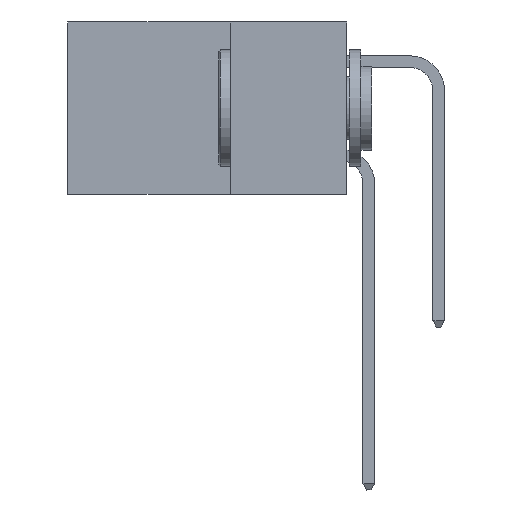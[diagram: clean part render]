
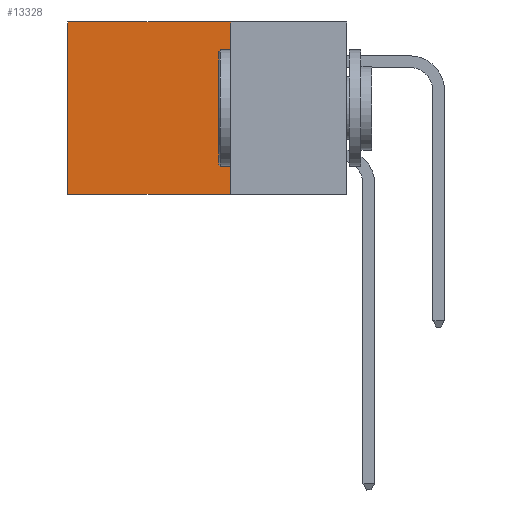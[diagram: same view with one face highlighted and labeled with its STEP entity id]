
A CAD part, left-side view. The second image highlights one B-rep face of the part: STEP entity #13328.
In plain terms, the highlighted planar face has unit normal (-1, 0, 0).
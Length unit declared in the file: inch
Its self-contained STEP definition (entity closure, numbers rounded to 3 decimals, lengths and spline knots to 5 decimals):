
#483 = ORIENTED_EDGE ( 'NONE', *, *, #14786, .F. ) ;
#1495 = CARTESIAN_POINT ( 'NONE',  ( 0.2875, 0.25, 0. ) ) ;
#2049 = ORIENTED_EDGE ( 'NONE', *, *, #6741, .F. ) ;
#3182 = CARTESIAN_POINT ( 'NONE',  ( 0.2875, 0.6, 0. ) ) ;
#3629 = DIRECTION ( 'NONE',  ( 0., 0., -1. ) ) ;
#5018 = VERTEX_POINT ( 'NONE', #12438 ) ;
#5411 = DIRECTION ( 'NONE',  ( 0., 0., -1. ) ) ;
#5612 = EDGE_LOOP ( 'NONE', ( #24950, #483, #2049, #9877 ) ) ;
#6403 = LINE ( 'NONE', #14993, #26133 ) ;
#6741 = EDGE_CURVE ( 'NONE', #13102, #5018, #8214, .T. ) ;
#6752 = DIRECTION ( 'NONE',  ( 0., 1., 0. ) ) ;
#8214 = LINE ( 'NONE', #10666, #30839 ) ;
#9877 = ORIENTED_EDGE ( 'NONE', *, *, #10642, .T. ) ;
#10642 = EDGE_CURVE ( 'NONE', #13102, #13510, #6403, .T. ) ;
#10666 = CARTESIAN_POINT ( 'NONE',  ( 0.2875, 0.25, 0. ) ) ;
#10961 = CARTESIAN_POINT ( 'NONE',  ( 0.2875, 0.6, -0.37 ) ) ;
#12245 = CARTESIAN_POINT ( 'NONE',  ( 0.2875, 0.25, 0. ) ) ;
#12438 = CARTESIAN_POINT ( 'NONE',  ( 0.2875, 0.25, -0.37 ) ) ;
#13102 = VERTEX_POINT ( 'NONE', #12245 ) ;
#13328 = ADVANCED_FACE ( 'NONE', ( #21765 ), #22157, .F. ) ;
#13510 = VERTEX_POINT ( 'NONE', #21050 ) ;
#13900 = DIRECTION ( 'NONE',  ( 1., 0., 0. ) ) ;
#13992 = VECTOR ( 'NONE', #24075, 39.37008 ) ;
#14786 = EDGE_CURVE ( 'NONE', #5018, #24750, #23316, .T. ) ;
#14993 = CARTESIAN_POINT ( 'NONE',  ( 0.2875, 0.25, 0. ) ) ;
#21050 = CARTESIAN_POINT ( 'NONE',  ( 0.2875, 0.6, 0. ) ) ;
#21234 = DIRECTION ( 'NONE',  ( 0., 0., -1. ) ) ;
#21765 = FACE_OUTER_BOUND ( 'NONE', #5612, .T. ) ;
#22157 = PLANE ( 'NONE',  #28763 ) ;
#23316 = LINE ( 'NONE', #31702, #13992 ) ;
#23651 = VECTOR ( 'NONE', #21234, 39.37008 ) ;
#24075 = DIRECTION ( 'NONE',  ( 0., 1., 0. ) ) ;
#24750 = VERTEX_POINT ( 'NONE', #10961 ) ;
#24950 = ORIENTED_EDGE ( 'NONE', *, *, #30598, .T. ) ;
#26133 = VECTOR ( 'NONE', #6752, 39.37008 ) ;
#28763 = AXIS2_PLACEMENT_3D ( 'NONE', #1495, #13900, #3629 ) ;
#30504 = LINE ( 'NONE', #3182, #23651 ) ;
#30598 = EDGE_CURVE ( 'NONE', #13510, #24750, #30504, .T. ) ;
#30839 = VECTOR ( 'NONE', #5411, 39.37008 ) ;
#31702 = CARTESIAN_POINT ( 'NONE',  ( 0.2875, 0.25, -0.37 ) ) ;
